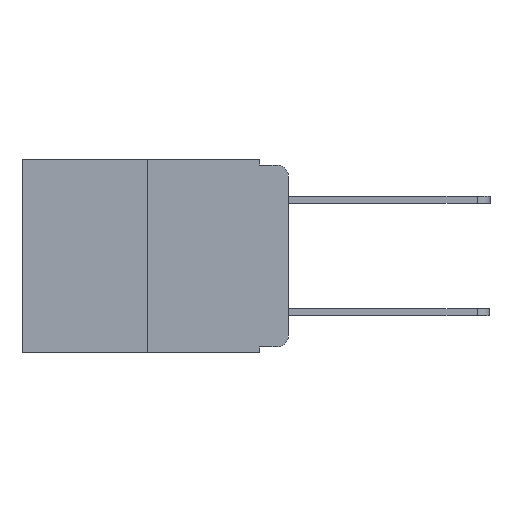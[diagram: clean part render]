
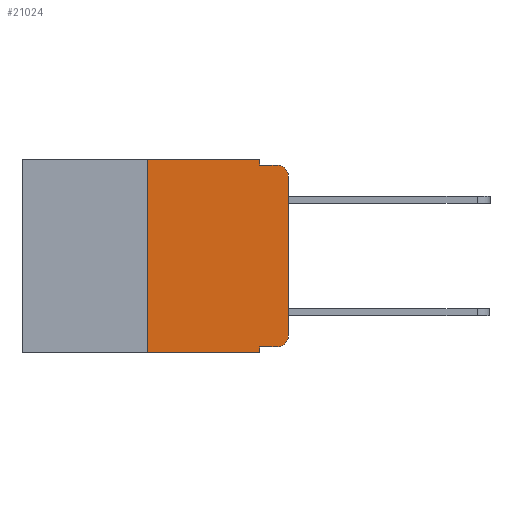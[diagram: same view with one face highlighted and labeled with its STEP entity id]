
A CAD part, left-side view. The second image highlights one B-rep face of the part: STEP entity #21024.
In plain terms, the highlighted planar face has unit normal (-1, 0, 0).
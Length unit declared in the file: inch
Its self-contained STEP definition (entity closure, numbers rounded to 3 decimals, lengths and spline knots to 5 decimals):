
#18 = CARTESIAN_POINT ( 'NONE',  ( 0., 0., 0. ) ) ;
#543 = CARTESIAN_POINT ( 'NONE',  ( 0., 0.051, -0.01 ) ) ;
#874 = DIRECTION ( 'NONE',  ( 0., 0., -1. ) ) ;
#915 = ORIENTED_EDGE ( 'NONE', *, *, #22359, .T. ) ;
#982 = VECTOR ( 'NONE', #7760, 39.37008 ) ;
#1071 = EDGE_CURVE ( 'NONE', #21979, #3038, #17427, .T. ) ;
#1093 = VERTEX_POINT ( 'NONE', #11324 ) ;
#1208 = VERTEX_POINT ( 'NONE', #21073 ) ;
#1214 = ORIENTED_EDGE ( 'NONE', *, *, #8628, .T. ) ;
#1225 = DIRECTION ( 'NONE',  ( 0., 0., -1. ) ) ;
#1367 = DIRECTION ( 'NONE',  ( 0., -1., 0. ) ) ;
#1616 = LINE ( 'NONE', #13263, #982 ) ;
#2321 = ORIENTED_EDGE ( 'NONE', *, *, #1071, .T. ) ;
#2560 = CARTESIAN_POINT ( 'NONE',  ( 0., 0.473, -0.343 ) ) ;
#2753 = DIRECTION ( 'NONE',  ( 0., 0., -1. ) ) ;
#3038 = VERTEX_POINT ( 'NONE', #17933 ) ;
#3367 = LINE ( 'NONE', #16482, #12250 ) ;
#3927 = EDGE_CURVE ( 'NONE', #21979, #1208, #7369, .T. ) ;
#4312 = DIRECTION ( 'NONE',  ( 0., -1., 0. ) ) ;
#5302 = CARTESIAN_POINT ( 'NONE',  ( 0., 0., -0.313 ) ) ;
#5452 = VERTEX_POINT ( 'NONE', #20394 ) ;
#5767 = CARTESIAN_POINT ( 'NONE',  ( 0., 0.25, 0. ) ) ;
#5870 = LINE ( 'NONE', #18, #10860 ) ;
#5902 = CARTESIAN_POINT ( 'NONE',  ( 0., 0.25, -0.343 ) ) ;
#6040 = EDGE_CURVE ( 'NONE', #1208, #22184, #21957, .T. ) ;
#6113 = DIRECTION ( 'NONE',  ( 0., -1., 0. ) ) ;
#7196 = VECTOR ( 'NONE', #14692, 39.37008 ) ;
#7369 = LINE ( 'NONE', #5767, #21553 ) ;
#7760 = DIRECTION ( 'NONE',  ( 0., 0., -1. ) ) ;
#7913 = LINE ( 'NONE', #15977, #22057 ) ;
#8032 = AXIS2_PLACEMENT_3D ( 'NONE', #10464, #12336, #874 ) ;
#8072 = CARTESIAN_POINT ( 'NONE',  ( 0., 0.02, -0.01 ) ) ;
#8122 = CARTESIAN_POINT ( 'NONE',  ( 0., 0.051, -0.333 ) ) ;
#8628 = EDGE_CURVE ( 'NONE', #5452, #9427, #24069, .T. ) ;
#9159 = VERTEX_POINT ( 'NONE', #5302 ) ;
#9427 = VERTEX_POINT ( 'NONE', #8072 ) ;
#9790 = ORIENTED_EDGE ( 'NONE', *, *, #6040, .F. ) ;
#10464 = CARTESIAN_POINT ( 'NONE',  ( 0., 0.473, 0. ) ) ;
#10663 = ORIENTED_EDGE ( 'NONE', *, *, #24306, .F. ) ;
#10860 = VECTOR ( 'NONE', #11506, 39.37008 ) ;
#11117 = VERTEX_POINT ( 'NONE', #543 ) ;
#11302 = CARTESIAN_POINT ( 'NONE',  ( 0., 0.02, -0.03 ) ) ;
#11324 = CARTESIAN_POINT ( 'NONE',  ( 0., 0.02, -0.333 ) ) ;
#11506 = DIRECTION ( 'NONE',  ( 0., 0., 1. ) ) ;
#12250 = VECTOR ( 'NONE', #1367, 39.37008 ) ;
#12336 = DIRECTION ( 'NONE',  ( 1., 0., 0. ) ) ;
#12412 = CARTESIAN_POINT ( 'NONE',  ( 0., 0.051, -0.333 ) ) ;
#12561 = LINE ( 'NONE', #8122, #21262 ) ;
#12661 = DIRECTION ( 'NONE',  ( -1., 0., 0. ) ) ;
#12829 = CARTESIAN_POINT ( 'NONE',  ( 0., 0.473, 0. ) ) ;
#13012 = ORIENTED_EDGE ( 'NONE', *, *, #18281, .T. ) ;
#13190 = DIRECTION ( 'NONE',  ( 0., 0., -1. ) ) ;
#13263 = CARTESIAN_POINT ( 'NONE',  ( 0., 0.051, 0. ) ) ;
#13855 = CARTESIAN_POINT ( 'NONE',  ( 0., 0.051, 0. ) ) ;
#13874 = FACE_OUTER_BOUND ( 'NONE', #21794, .T. ) ;
#13987 = CIRCLE ( 'NONE', #14643, 0.02 ) ;
#14643 = AXIS2_PLACEMENT_3D ( 'NONE', #23679, #12661, #1225 ) ;
#14692 = DIRECTION ( 'NONE',  ( 0., -1., 0. ) ) ;
#15310 = EDGE_CURVE ( 'NONE', #22184, #11117, #1616, .T. ) ;
#15977 = CARTESIAN_POINT ( 'NONE',  ( 0., 0.051, 0. ) ) ;
#16482 = CARTESIAN_POINT ( 'NONE',  ( 0., 0.051, -0.01 ) ) ;
#16531 = ORIENTED_EDGE ( 'NONE', *, *, #23145, .T. ) ;
#17427 = LINE ( 'NONE', #2560, #21686 ) ;
#17933 = CARTESIAN_POINT ( 'NONE',  ( 0., 0.051, -0.343 ) ) ;
#18271 = ORIENTED_EDGE ( 'NONE', *, *, #3927, .F. ) ;
#18281 = EDGE_CURVE ( 'NONE', #1093, #9159, #13987, .T. ) ;
#18441 = AXIS2_PLACEMENT_3D ( 'NONE', #11302, #24163, #13190 ) ;
#18860 = DIRECTION ( 'NONE',  ( 0., 0., 1. ) ) ;
#20394 = CARTESIAN_POINT ( 'NONE',  ( 0., 0., -0.03 ) ) ;
#20809 = ORIENTED_EDGE ( 'NONE', *, *, #15310, .F. ) ;
#21024 = ADVANCED_FACE ( 'NONE', ( #13874 ), #21556, .F. ) ;
#21057 = VERTEX_POINT ( 'NONE', #12412 ) ;
#21073 = CARTESIAN_POINT ( 'NONE',  ( 0., 0.25, 0. ) ) ;
#21262 = VECTOR ( 'NONE', #4312, 39.37008 ) ;
#21553 = VECTOR ( 'NONE', #18860, 39.37008 ) ;
#21556 = PLANE ( 'NONE',  #8032 ) ;
#21686 = VECTOR ( 'NONE', #6113, 39.37008 ) ;
#21794 = EDGE_LOOP ( 'NONE', ( #915, #1214, #23783, #20809, #9790, #18271, #2321, #10663, #16531, #13012 ) ) ;
#21957 = LINE ( 'NONE', #12829, #7196 ) ;
#21979 = VERTEX_POINT ( 'NONE', #5902 ) ;
#22057 = VECTOR ( 'NONE', #2753, 39.37008 ) ;
#22184 = VERTEX_POINT ( 'NONE', #13855 ) ;
#22359 = EDGE_CURVE ( 'NONE', #9159, #5452, #5870, .T. ) ;
#23145 = EDGE_CURVE ( 'NONE', #21057, #1093, #12561, .T. ) ;
#23679 = CARTESIAN_POINT ( 'NONE',  ( 0., 0.02, -0.313 ) ) ;
#23783 = ORIENTED_EDGE ( 'NONE', *, *, #23875, .F. ) ;
#23875 = EDGE_CURVE ( 'NONE', #11117, #9427, #3367, .T. ) ;
#24069 = CIRCLE ( 'NONE', #18441, 0.02 ) ;
#24163 = DIRECTION ( 'NONE',  ( -1., 0., 0. ) ) ;
#24306 = EDGE_CURVE ( 'NONE', #21057, #3038, #7913, .T. ) ;
